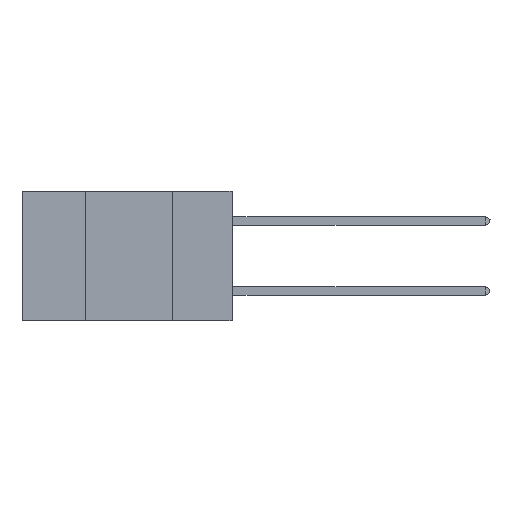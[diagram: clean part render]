
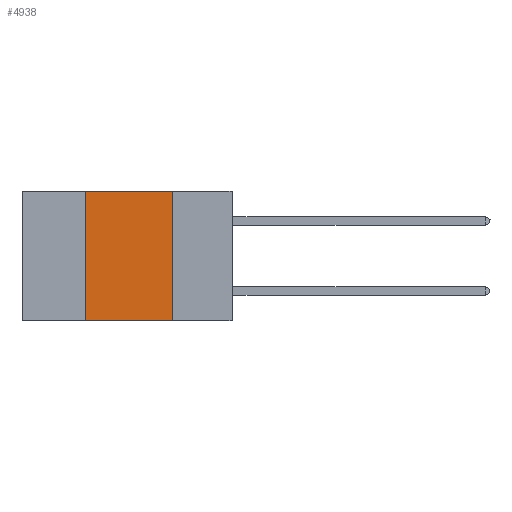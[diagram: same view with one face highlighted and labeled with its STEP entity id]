
A CAD part, left-side view. The second image highlights one B-rep face of the part: STEP entity #4938.
In plain terms, the highlighted planar face has unit normal (-1, 0, 0).
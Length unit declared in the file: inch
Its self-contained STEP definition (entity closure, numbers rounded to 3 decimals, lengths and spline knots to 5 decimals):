
#121 = DIRECTION ( 'NONE',  ( 0., -1., 0. ) ) ;
#418 = ORIENTED_EDGE ( 'NONE', *, *, #4880, .F. ) ;
#993 = DIRECTION ( 'NONE',  ( 0., 0., -1. ) ) ;
#1249 = ORIENTED_EDGE ( 'NONE', *, *, #8814, .T. ) ;
#1371 = FACE_OUTER_BOUND ( 'NONE', #16304, .T. ) ;
#1475 = LINE ( 'NONE', #7698, #12584 ) ;
#2665 = ORIENTED_EDGE ( 'NONE', *, *, #13711, .F. ) ;
#3224 = CARTESIAN_POINT ( 'NONE',  ( 0., 0.17, 0. ) ) ;
#3360 = LINE ( 'NONE', #13482, #12065 ) ;
#3908 = CARTESIAN_POINT ( 'NONE',  ( 0., 0.42, 0. ) ) ;
#4695 = DIRECTION ( 'NONE',  ( 0., 0., -1. ) ) ;
#4880 = EDGE_CURVE ( 'NONE', #15918, #5821, #12846, .T. ) ;
#4938 = ADVANCED_FACE ( 'NONE', ( #1371 ), #6599, .F. ) ;
#5765 = CARTESIAN_POINT ( 'NONE',  ( 0., 0.17, -0.37 ) ) ;
#5821 = VERTEX_POINT ( 'NONE', #3224 ) ;
#6448 = CARTESIAN_POINT ( 'NONE',  ( 0., 0.6, 0. ) ) ;
#6599 = PLANE ( 'NONE',  #12192 ) ;
#7059 = VERTEX_POINT ( 'NONE', #15712 ) ;
#7428 = VECTOR ( 'NONE', #121, 39.37008 ) ;
#7698 = CARTESIAN_POINT ( 'NONE',  ( 0., 0.42, 0. ) ) ;
#7855 = DIRECTION ( 'NONE',  ( 1., 0., 0. ) ) ;
#7947 = LINE ( 'NONE', #12946, #13847 ) ;
#8814 = EDGE_CURVE ( 'NONE', #7059, #13705, #7947, .T. ) ;
#12065 = VECTOR ( 'NONE', #4695, 39.37008 ) ;
#12192 = AXIS2_PLACEMENT_3D ( 'NONE', #6448, #7855, #993 ) ;
#12531 = DIRECTION ( 'NONE',  ( 0., 0., 1. ) ) ;
#12584 = VECTOR ( 'NONE', #12531, 39.37008 ) ;
#12846 = LINE ( 'NONE', #14001, #7428 ) ;
#12934 = ORIENTED_EDGE ( 'NONE', *, *, #13016, .F. ) ;
#12946 = CARTESIAN_POINT ( 'NONE',  ( 0., 0.6, -0.37 ) ) ;
#13016 = EDGE_CURVE ( 'NONE', #7059, #15918, #1475, .T. ) ;
#13482 = CARTESIAN_POINT ( 'NONE',  ( 0., 0.17, 0. ) ) ;
#13705 = VERTEX_POINT ( 'NONE', #5765 ) ;
#13711 = EDGE_CURVE ( 'NONE', #5821, #13705, #3360, .T. ) ;
#13847 = VECTOR ( 'NONE', #14506, 39.37008 ) ;
#14001 = CARTESIAN_POINT ( 'NONE',  ( 0., 0.6, 0. ) ) ;
#14506 = DIRECTION ( 'NONE',  ( 0., -1., 0. ) ) ;
#15712 = CARTESIAN_POINT ( 'NONE',  ( 0., 0.42, -0.37 ) ) ;
#15918 = VERTEX_POINT ( 'NONE', #3908 ) ;
#16304 = EDGE_LOOP ( 'NONE', ( #2665, #418, #12934, #1249 ) ) ;
